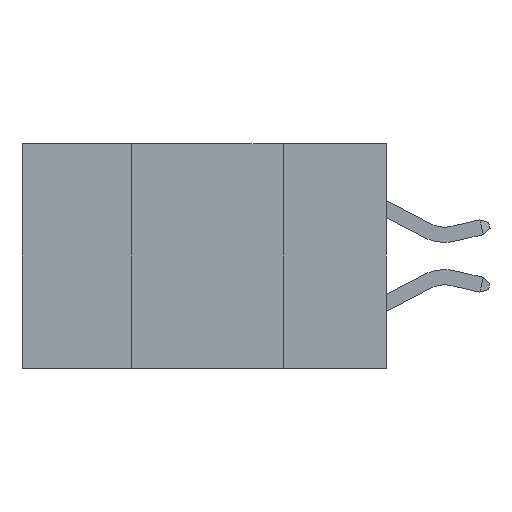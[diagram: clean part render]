
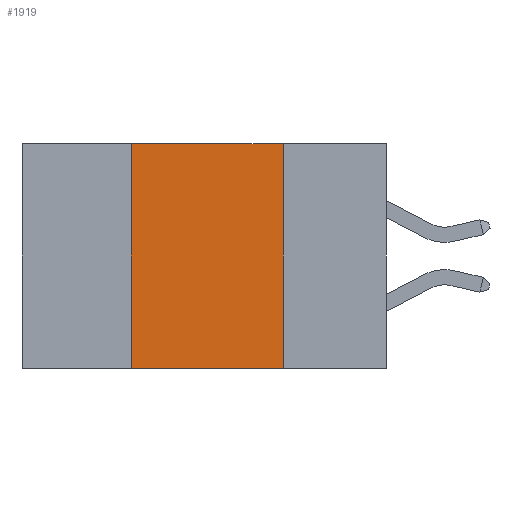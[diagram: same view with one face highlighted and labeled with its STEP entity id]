
A CAD part, left-side view. The second image highlights one B-rep face of the part: STEP entity #1919.
In plain terms, the highlighted planar face has unit normal (-1, 0, 0).
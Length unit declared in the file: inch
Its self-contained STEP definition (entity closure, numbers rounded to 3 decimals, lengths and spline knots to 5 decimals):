
#564 = CARTESIAN_POINT ( 'NONE',  ( 0., 0.6, -0.37 ) ) ;
#1055 = ORIENTED_EDGE ( 'NONE', *, *, #21515, .F. ) ;
#1919 = ADVANCED_FACE ( 'NONE', ( #10638 ), #14145, .F. ) ;
#2552 = LINE ( 'NONE', #11080, #16188 ) ;
#3287 = DIRECTION ( 'NONE',  ( 0., 0., -1. ) ) ;
#3398 = VECTOR ( 'NONE', #9435, 39.37008 ) ;
#3765 = VERTEX_POINT ( 'NONE', #4157 ) ;
#3775 = VERTEX_POINT ( 'NONE', #7731 ) ;
#4157 = CARTESIAN_POINT ( 'NONE',  ( 0., 0.42, 0. ) ) ;
#5056 = DIRECTION ( 'NONE',  ( 1., 0., 0. ) ) ;
#7731 = CARTESIAN_POINT ( 'NONE',  ( 0., 0.42, -0.37 ) ) ;
#8060 = EDGE_CURVE ( 'NONE', #3765, #21338, #15697, .T. ) ;
#9435 = DIRECTION ( 'NONE',  ( 0., 0., -1. ) ) ;
#10638 = FACE_OUTER_BOUND ( 'NONE', #14929, .T. ) ;
#10694 = EDGE_CURVE ( 'NONE', #3775, #16282, #19278, .T. ) ;
#10928 = DIRECTION ( 'NONE',  ( 0., 0., 1. ) ) ;
#11080 = CARTESIAN_POINT ( 'NONE',  ( 0., 0.42, 0. ) ) ;
#11709 = CARTESIAN_POINT ( 'NONE',  ( 0., 0.17, -0.37 ) ) ;
#13162 = ORIENTED_EDGE ( 'NONE', *, *, #8060, .F. ) ;
#14145 = PLANE ( 'NONE',  #22930 ) ;
#14760 = ORIENTED_EDGE ( 'NONE', *, *, #21970, .F. ) ;
#14824 = ORIENTED_EDGE ( 'NONE', *, *, #10694, .T. ) ;
#14929 = EDGE_LOOP ( 'NONE', ( #1055, #13162, #14760, #14824 ) ) ;
#15697 = LINE ( 'NONE', #23008, #16523 ) ;
#16188 = VECTOR ( 'NONE', #10928, 39.37008 ) ;
#16282 = VERTEX_POINT ( 'NONE', #11709 ) ;
#16523 = VECTOR ( 'NONE', #21274, 39.37008 ) ;
#18278 = DIRECTION ( 'NONE',  ( 0., -1., 0. ) ) ;
#19278 = LINE ( 'NONE', #564, #21504 ) ;
#19330 = LINE ( 'NONE', #20170, #3398 ) ;
#20170 = CARTESIAN_POINT ( 'NONE',  ( 0., 0.17, 0. ) ) ;
#21274 = DIRECTION ( 'NONE',  ( 0., -1., 0. ) ) ;
#21338 = VERTEX_POINT ( 'NONE', #22019 ) ;
#21504 = VECTOR ( 'NONE', #18278, 39.37008 ) ;
#21515 = EDGE_CURVE ( 'NONE', #21338, #16282, #19330, .T. ) ;
#21970 = EDGE_CURVE ( 'NONE', #3775, #3765, #2552, .T. ) ;
#22019 = CARTESIAN_POINT ( 'NONE',  ( 0., 0.17, 0. ) ) ;
#22930 = AXIS2_PLACEMENT_3D ( 'NONE', #23116, #5056, #3287 ) ;
#23008 = CARTESIAN_POINT ( 'NONE',  ( 0., 0.6, 0. ) ) ;
#23116 = CARTESIAN_POINT ( 'NONE',  ( 0., 0.6, 0. ) ) ;
